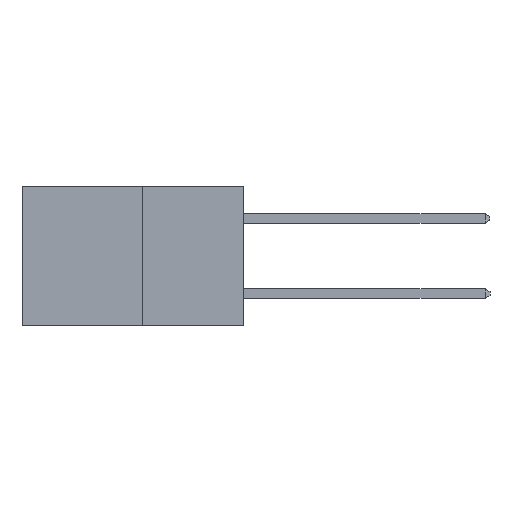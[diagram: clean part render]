
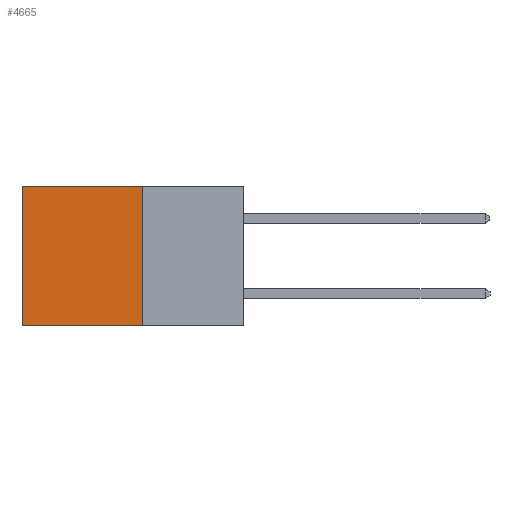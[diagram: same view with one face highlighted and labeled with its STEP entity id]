
A CAD part, left-side view. The second image highlights one B-rep face of the part: STEP entity #4665.
In plain terms, the highlighted planar face has unit normal (-1, 0, 0).
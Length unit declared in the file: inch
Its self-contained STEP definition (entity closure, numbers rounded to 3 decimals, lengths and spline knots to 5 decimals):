
#33 = CARTESIAN_POINT ( 'NONE',  ( 0.277, 0.27, -0.37 ) ) ;
#398 = DIRECTION ( 'NONE',  ( 0., 1., 0. ) ) ;
#565 = ORIENTED_EDGE ( 'NONE', *, *, #4014, .T. ) ;
#856 = LINE ( 'NONE', #4331, #4355 ) ;
#1314 = VERTEX_POINT ( 'NONE', #3343 ) ;
#1449 = VERTEX_POINT ( 'NONE', #6941 ) ;
#1730 = FACE_OUTER_BOUND ( 'NONE', #7669, .T. ) ;
#1939 = VECTOR ( 'NONE', #398, 39.37008 ) ;
#2041 = CARTESIAN_POINT ( 'NONE',  ( 0.277, 0.27, 0. ) ) ;
#2061 = CARTESIAN_POINT ( 'NONE',  ( 0.277, 0.27, -0.37 ) ) ;
#2273 = VECTOR ( 'NONE', #5685, 39.37008 ) ;
#2521 = LINE ( 'NONE', #2061, #8770 ) ;
#2811 = DIRECTION ( 'NONE',  ( 0., 0., -1. ) ) ;
#2872 = ORIENTED_EDGE ( 'NONE', *, *, #2919, .F. ) ;
#2919 = EDGE_CURVE ( 'NONE', #6073, #8111, #2521, .T. ) ;
#3343 = CARTESIAN_POINT ( 'NONE',  ( 0.277, 0.59, -0.37 ) ) ;
#3738 = EDGE_CURVE ( 'NONE', #1449, #1314, #4145, .T. ) ;
#3887 = CARTESIAN_POINT ( 'NONE',  ( 0.277, 0.27, 0. ) ) ;
#4014 = EDGE_CURVE ( 'NONE', #6073, #1449, #5652, .T. ) ;
#4145 = LINE ( 'NONE', #7684, #2273 ) ;
#4251 = ORIENTED_EDGE ( 'NONE', *, *, #3738, .T. ) ;
#4331 = CARTESIAN_POINT ( 'NONE',  ( 0.277, 0.27, -0.37 ) ) ;
#4355 = VECTOR ( 'NONE', #5035, 39.37008 ) ;
#4665 = ADVANCED_FACE ( 'NONE', ( #1730 ), #5553, .F. ) ;
#4881 = ORIENTED_EDGE ( 'NONE', *, *, #5201, .F. ) ;
#5035 = DIRECTION ( 'NONE',  ( 0., 1., 0. ) ) ;
#5201 = EDGE_CURVE ( 'NONE', #8111, #1314, #856, .T. ) ;
#5553 = PLANE ( 'NONE',  #7126 ) ;
#5652 = LINE ( 'NONE', #3887, #1939 ) ;
#5685 = DIRECTION ( 'NONE',  ( 0., 0., -1. ) ) ;
#6073 = VERTEX_POINT ( 'NONE', #2041 ) ;
#6233 = DIRECTION ( 'NONE',  ( 0., 0., -1. ) ) ;
#6941 = CARTESIAN_POINT ( 'NONE',  ( 0.277, 0.59, 0. ) ) ;
#6958 = DIRECTION ( 'NONE',  ( 1., 0., 0. ) ) ;
#7126 = AXIS2_PLACEMENT_3D ( 'NONE', #33, #6958, #2811 ) ;
#7669 = EDGE_LOOP ( 'NONE', ( #4251, #4881, #2872, #565 ) ) ;
#7684 = CARTESIAN_POINT ( 'NONE',  ( 0.277, 0.59, -0.37 ) ) ;
#8111 = VERTEX_POINT ( 'NONE', #8619 ) ;
#8619 = CARTESIAN_POINT ( 'NONE',  ( 0.277, 0.27, -0.37 ) ) ;
#8770 = VECTOR ( 'NONE', #6233, 39.37008 ) ;
